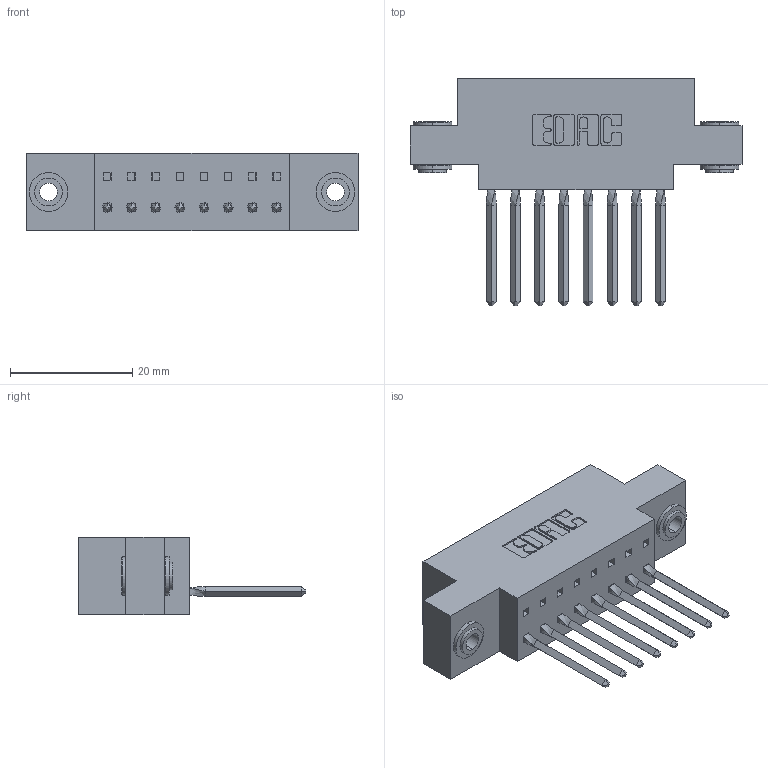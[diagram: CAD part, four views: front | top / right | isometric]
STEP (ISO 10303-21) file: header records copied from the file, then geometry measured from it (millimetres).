
FILE_DESCRIPTION (( 'STEP AP203' ), '1' );
FILE_NAME ('317-008-541-603.STEP', '2020-02-27T13:09:03', ( '' ), ( '' ), 'SwSTEP 2.0', 'SolidWorks 2016', '' );
FILE_SCHEMA (( 'CONFIG_CONTROL_DESIGN' ));
Length unit declared in the file: inch
Products named in the file (4): 317-290-002_541; 317-008-541-603; 317 Part_.156 Dia - TH; 345-250-002_345-250-002-102
Assembly tree (11 placements, depth 2):
  317-008-541-603
    317 Part_.156 Dia - TH
    317-290-002_541  x8
    345-250-002_345-250-002-102  x2
Bounding box: 54.41 x 37.34 x 12.7 mm (x, y, z)
Volume: 7796.9 mm3; surface area: 10098.7 mm2
Topology: 11 solids, 11 shells, 1356 faces, 3823 edges, 2486 vertices
Faces by surface type: plane 1060, cylinder 256, bspline 32, cone 8
Entity records: 18249 total; most frequent: CARTESIAN_POINT 3836, ORIENTED_EDGE 3090, DIRECTION 2555, EDGE_CURVE 1545, LINE 1157, VECTOR 1157, VERTEX_POINT 1020, AXIS2_PLACEMENT_3D 699
